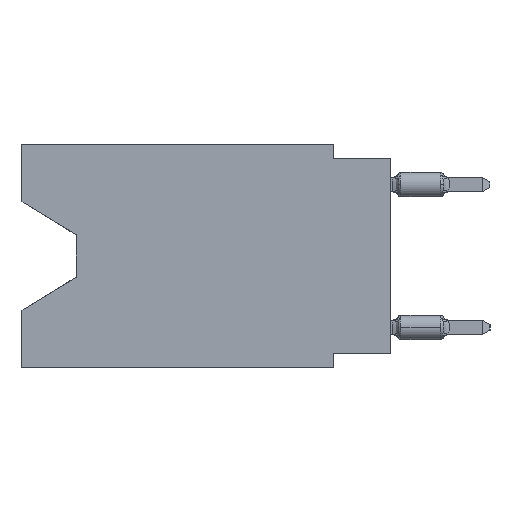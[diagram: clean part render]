
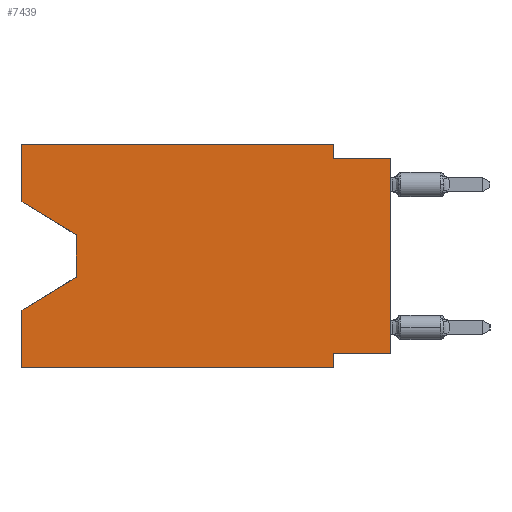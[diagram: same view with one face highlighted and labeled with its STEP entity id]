
A CAD part, left-side view. The second image highlights one B-rep face of the part: STEP entity #7439.
In plain terms, the highlighted planar face has unit normal (-1, 0, 0).
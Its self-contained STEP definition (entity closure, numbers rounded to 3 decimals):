
#277 = LINE ( 'NONE', #6145, #14523 ) ;
#1031 = CARTESIAN_POINT ( 'NONE',  ( 0., 2.54, -0.635 ) ) ;
#1438 = VECTOR ( 'NONE', #26544, 1000. ) ;
#2761 = ORIENTED_EDGE ( 'NONE', *, *, #24016, .F. ) ;
#3135 = DIRECTION ( 'NONE',  ( 0., 0., -1. ) ) ;
#3301 = VERTEX_POINT ( 'NONE', #31449 ) ;
#4061 = VERTEX_POINT ( 'NONE', #46727 ) ;
#4446 = ORIENTED_EDGE ( 'NONE', *, *, #5072, .T. ) ;
#4899 = ORIENTED_EDGE ( 'NONE', *, *, #60931, .F. ) ;
#5072 = EDGE_CURVE ( 'NONE', #9265, #63810, #59286, .T. ) ;
#5931 = CARTESIAN_POINT ( 'NONE',  ( 0., 16.383, -2.546 ) ) ;
#6145 = CARTESIAN_POINT ( 'NONE',  ( 0., 0., 0. ) ) ;
#6874 = CARTESIAN_POINT ( 'NONE',  ( 0., 16.383, 0. ) ) ;
#7439 = ADVANCED_FACE ( 'NONE', ( #42105 ), #28302, .F. ) ;
#8181 = VECTOR ( 'NONE', #14536, 1000. ) ;
#8461 = CARTESIAN_POINT ( 'NONE',  ( 0., 16.383, -2.546 ) ) ;
#8677 = LINE ( 'NONE', #43798, #8181 ) ;
#9265 = VERTEX_POINT ( 'NONE', #18738 ) ;
#9584 = CARTESIAN_POINT ( 'NONE',  ( 0., 0., -0.635 ) ) ;
#9988 = ORIENTED_EDGE ( 'NONE', *, *, #64209, .F. ) ;
#11911 = DIRECTION ( 'NONE',  ( 0., 0., -1. ) ) ;
#12890 = LINE ( 'NONE', #38196, #49348 ) ;
#13000 = EDGE_CURVE ( 'NONE', #52457, #39923, #12890, .T. ) ;
#14523 = VECTOR ( 'NONE', #35676, 1000. ) ;
#14536 = DIRECTION ( 'NONE',  ( 0., 0., 1. ) ) ;
#14591 = CARTESIAN_POINT ( 'NONE',  ( 0., 16.383, -9.906 ) ) ;
#15001 = CARTESIAN_POINT ( 'NONE',  ( 0., 13.97, -5.893 ) ) ;
#15484 = ORIENTED_EDGE ( 'NONE', *, *, #33223, .F. ) ;
#15587 = CARTESIAN_POINT ( 'NONE',  ( 0., 13.97, -4.013 ) ) ;
#16526 = VECTOR ( 'NONE', #3135, 1000. ) ;
#17285 = CARTESIAN_POINT ( 'NONE',  ( 0., 0., -0.635 ) ) ;
#17613 = LINE ( 'NONE', #17285, #33320 ) ;
#18598 = DIRECTION ( 'NONE',  ( 0., -1., 0. ) ) ;
#18738 = CARTESIAN_POINT ( 'NONE',  ( 0., 16.383, -9.906 ) ) ;
#19386 = CARTESIAN_POINT ( 'NONE',  ( 0., 0., -9.271 ) ) ;
#20534 = LINE ( 'NONE', #15587, #16526 ) ;
#21238 = VECTOR ( 'NONE', #41236, 1000. ) ;
#22124 = ORIENTED_EDGE ( 'NONE', *, *, #33361, .F. ) ;
#24016 = EDGE_CURVE ( 'NONE', #9265, #46203, #8677, .T. ) ;
#25174 = LINE ( 'NONE', #15001, #62774 ) ;
#26544 = DIRECTION ( 'NONE',  ( 0., 0., 1. ) ) ;
#27234 = VERTEX_POINT ( 'NONE', #29246 ) ;
#27914 = CARTESIAN_POINT ( 'NONE',  ( 0., 16.383, -7.36 ) ) ;
#28302 = PLANE ( 'NONE',  #49792 ) ;
#29246 = CARTESIAN_POINT ( 'NONE',  ( 0., 16.383, 0. ) ) ;
#29262 = VECTOR ( 'NONE', #48957, 1000. ) ;
#30021 = DIRECTION ( 'NONE',  ( 0., -1., 0. ) ) ;
#31449 = CARTESIAN_POINT ( 'NONE',  ( 0., 13.97, -4.013 ) ) ;
#32586 = DIRECTION ( 'NONE',  ( 1., 0., 0. ) ) ;
#33058 = CARTESIAN_POINT ( 'NONE',  ( 0., 0., -9.271 ) ) ;
#33223 = EDGE_CURVE ( 'NONE', #27234, #52457, #37977, .T. ) ;
#33320 = VECTOR ( 'NONE', #38309, 1000. ) ;
#33361 = EDGE_CURVE ( 'NONE', #39923, #45832, #17613, .T. ) ;
#33577 = EDGE_LOOP ( 'NONE', ( #53465, #60579, #40860, #2761, #4446, #55058, #4899, #54622, #22124, #49218, #15484, #9988 ) ) ;
#35676 = DIRECTION ( 'NONE',  ( 0., 0., 1. ) ) ;
#35776 = LINE ( 'NONE', #6874, #1438 ) ;
#36266 = EDGE_CURVE ( 'NONE', #4061, #46203, #25174, .T. ) ;
#37206 = DIRECTION ( 'NONE',  ( 0., 0., -1. ) ) ;
#37977 = LINE ( 'NONE', #42554, #55292 ) ;
#38196 = CARTESIAN_POINT ( 'NONE',  ( 0., 2.54, 0. ) ) ;
#38309 = DIRECTION ( 'NONE',  ( 0., -1., 0. ) ) ;
#39923 = VERTEX_POINT ( 'NONE', #1031 ) ;
#40760 = EDGE_CURVE ( 'NONE', #3301, #4061, #20534, .T. ) ;
#40860 = ORIENTED_EDGE ( 'NONE', *, *, #36266, .T. ) ;
#41236 = DIRECTION ( 'NONE',  ( 0., 0., -1. ) ) ;
#42105 = FACE_OUTER_BOUND ( 'NONE', #33577, .T. ) ;
#42554 = CARTESIAN_POINT ( 'NONE',  ( 0., 16.383, 0. ) ) ;
#43798 = CARTESIAN_POINT ( 'NONE',  ( 0., 16.383, 0. ) ) ;
#44417 = CARTESIAN_POINT ( 'NONE',  ( 0., 2.54, -9.906 ) ) ;
#45832 = VERTEX_POINT ( 'NONE', #9584 ) ;
#46168 = LINE ( 'NONE', #47152, #21238 ) ;
#46203 = VERTEX_POINT ( 'NONE', #27914 ) ;
#46727 = CARTESIAN_POINT ( 'NONE',  ( 0., 13.97, -5.893 ) ) ;
#46963 = EDGE_CURVE ( 'NONE', #52223, #63810, #46168, .T. ) ;
#47152 = CARTESIAN_POINT ( 'NONE',  ( 0., 2.54, -9.906 ) ) ;
#47546 = VECTOR ( 'NONE', #30021, 1000. ) ;
#48360 = CARTESIAN_POINT ( 'NONE',  ( 0., 16.383, 0. ) ) ;
#48957 = DIRECTION ( 'NONE',  ( 0., 1., 0. ) ) ;
#49201 = DIRECTION ( 'NONE',  ( 0., 0.855, -0.519 ) ) ;
#49218 = ORIENTED_EDGE ( 'NONE', *, *, #13000, .F. ) ;
#49348 = VECTOR ( 'NONE', #11911, 1000. ) ;
#49792 = AXIS2_PLACEMENT_3D ( 'NONE', #48360, #32586, #37206 ) ;
#52223 = VERTEX_POINT ( 'NONE', #64601 ) ;
#52457 = VERTEX_POINT ( 'NONE', #61944 ) ;
#52528 = VERTEX_POINT ( 'NONE', #33058 ) ;
#53089 = EDGE_CURVE ( 'NONE', #54512, #3301, #55181, .T. ) ;
#53465 = ORIENTED_EDGE ( 'NONE', *, *, #53089, .T. ) ;
#54512 = VERTEX_POINT ( 'NONE', #8461 ) ;
#54622 = ORIENTED_EDGE ( 'NONE', *, *, #60205, .T. ) ;
#55058 = ORIENTED_EDGE ( 'NONE', *, *, #46963, .F. ) ;
#55181 = LINE ( 'NONE', #5931, #58074 ) ;
#55292 = VECTOR ( 'NONE', #18598, 1000. ) ;
#58074 = VECTOR ( 'NONE', #61062, 1000. ) ;
#59286 = LINE ( 'NONE', #14591, #47546 ) ;
#60205 = EDGE_CURVE ( 'NONE', #52528, #45832, #277, .T. ) ;
#60579 = ORIENTED_EDGE ( 'NONE', *, *, #40760, .T. ) ;
#60931 = EDGE_CURVE ( 'NONE', #52528, #52223, #64358, .T. ) ;
#61062 = DIRECTION ( 'NONE',  ( 0., -0.855, -0.519 ) ) ;
#61944 = CARTESIAN_POINT ( 'NONE',  ( 0., 2.54, 0. ) ) ;
#62774 = VECTOR ( 'NONE', #49201, 1000. ) ;
#63810 = VERTEX_POINT ( 'NONE', #44417 ) ;
#64209 = EDGE_CURVE ( 'NONE', #54512, #27234, #35776, .T. ) ;
#64358 = LINE ( 'NONE', #19386, #29262 ) ;
#64601 = CARTESIAN_POINT ( 'NONE',  ( 0., 2.54, -9.271 ) ) ;
